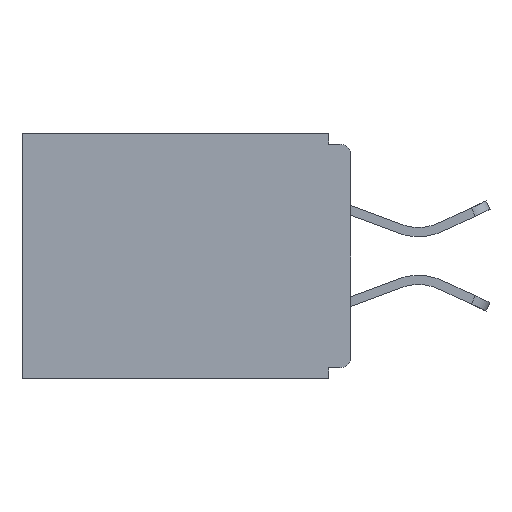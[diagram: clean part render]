
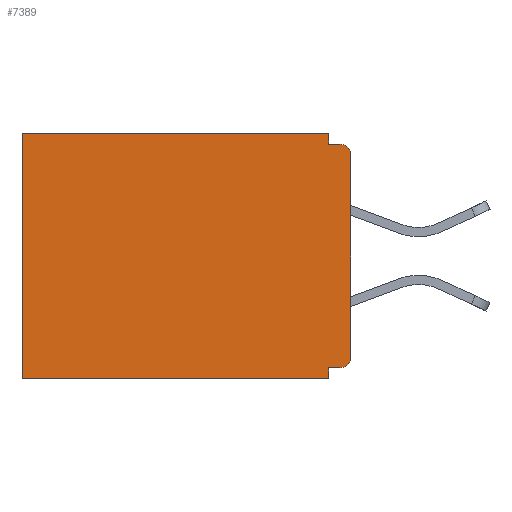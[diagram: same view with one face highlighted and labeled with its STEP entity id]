
A CAD part, left-side view. The second image highlights one B-rep face of the part: STEP entity #7389.
In plain terms, the highlighted planar face has unit normal (-1, 0, 0).
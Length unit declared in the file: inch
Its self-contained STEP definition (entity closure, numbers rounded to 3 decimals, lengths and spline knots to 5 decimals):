
#33 = ORIENTED_EDGE ( 'NONE', *, *, #11274, .F. ) ;
#66 = VECTOR ( 'NONE', #2666, 39.37008 ) ;
#391 = LINE ( 'NONE', #12094, #10864 ) ;
#463 = VECTOR ( 'NONE', #8896, 39.37008 ) ;
#676 = VERTEX_POINT ( 'NONE', #4409 ) ;
#1182 = VECTOR ( 'NONE', #12163, 39.37008 ) ;
#1606 = EDGE_CURVE ( 'NONE', #3405, #9363, #13358, .T. ) ;
#1811 = VECTOR ( 'NONE', #3227, 39.37008 ) ;
#2247 = LINE ( 'NONE', #7688, #2940 ) ;
#2350 = LINE ( 'NONE', #8434, #66 ) ;
#2666 = DIRECTION ( 'NONE',  ( 0., 1., 0. ) ) ;
#2933 = VERTEX_POINT ( 'NONE', #11107 ) ;
#2940 = VECTOR ( 'NONE', #10080, 39.37008 ) ;
#2948 = VERTEX_POINT ( 'NONE', #11156 ) ;
#2964 = ORIENTED_EDGE ( 'NONE', *, *, #5777, .T. ) ;
#3064 = DIRECTION ( 'NONE',  ( -1., 0., 0. ) ) ;
#3100 = ORIENTED_EDGE ( 'NONE', *, *, #1606, .F. ) ;
#3113 = ORIENTED_EDGE ( 'NONE', *, *, #5109, .T. ) ;
#3227 = DIRECTION ( 'NONE',  ( 0., 0., -1. ) ) ;
#3266 = CIRCLE ( 'NONE', #5534, 0.015 ) ;
#3405 = VERTEX_POINT ( 'NONE', #8879 ) ;
#3455 = VECTOR ( 'NONE', #6481, 39.37008 ) ;
#4177 = CARTESIAN_POINT ( 'NONE',  ( 0.298, 0., -0.015 ) ) ;
#4213 = DIRECTION ( 'NONE',  ( 0., 0., -1. ) ) ;
#4240 = AXIS2_PLACEMENT_3D ( 'NONE', #8435, #9583, #4910 ) ;
#4270 = CARTESIAN_POINT ( 'NONE',  ( 0.298, 0.031, -0.343 ) ) ;
#4409 = CARTESIAN_POINT ( 'NONE',  ( 0.298, 0.031, -0.343 ) ) ;
#4434 = ORIENTED_EDGE ( 'NONE', *, *, #14666, .F. ) ;
#4571 = VERTEX_POINT ( 'NONE', #10166 ) ;
#4628 = FACE_OUTER_BOUND ( 'NONE', #9321, .T. ) ;
#4910 = DIRECTION ( 'NONE',  ( 0., 0., -1. ) ) ;
#5109 = EDGE_CURVE ( 'NONE', #2948, #9160, #5795, .T. ) ;
#5123 = CARTESIAN_POINT ( 'NONE',  ( 0.298, 0.46, 0. ) ) ;
#5504 = CARTESIAN_POINT ( 'NONE',  ( 0.298, 0., -0.313 ) ) ;
#5534 = AXIS2_PLACEMENT_3D ( 'NONE', #9932, #3064, #4213 ) ;
#5617 = EDGE_CURVE ( 'NONE', #10846, #2948, #6871, .T. ) ;
#5777 = EDGE_CURVE ( 'NONE', #13731, #9363, #3266, .T. ) ;
#5795 = LINE ( 'NONE', #5123, #13452 ) ;
#5915 = CARTESIAN_POINT ( 'NONE',  ( 0.298, 0.015, -0.328 ) ) ;
#6049 = AXIS2_PLACEMENT_3D ( 'NONE', #11070, #7735, #7685 ) ;
#6290 = DIRECTION ( 'NONE',  ( 0., 0., -1. ) ) ;
#6481 = DIRECTION ( 'NONE',  ( 0., 0., -1. ) ) ;
#6674 = PLANE ( 'NONE',  #6049 ) ;
#6854 = CARTESIAN_POINT ( 'NONE',  ( 0.298, 0.46, -0.343 ) ) ;
#6871 = LINE ( 'NONE', #8862, #463 ) ;
#7298 = EDGE_CURVE ( 'NONE', #3405, #11659, #10030, .T. ) ;
#7389 = ADVANCED_FACE ( 'NONE', ( #4628 ), #6674, .F. ) ;
#7685 = DIRECTION ( 'NONE',  ( 0., 0., -1. ) ) ;
#7688 = CARTESIAN_POINT ( 'NONE',  ( 0.298, 0.031, -0.343 ) ) ;
#7735 = DIRECTION ( 'NONE',  ( 1., 0., 0. ) ) ;
#8434 = CARTESIAN_POINT ( 'NONE',  ( 0.298, 0., -0.343 ) ) ;
#8435 = CARTESIAN_POINT ( 'NONE',  ( 0.298, 0.015, -0.03 ) ) ;
#8682 = LINE ( 'NONE', #4177, #1182 ) ;
#8862 = CARTESIAN_POINT ( 'NONE',  ( 0.298, 0., 0. ) ) ;
#8879 = CARTESIAN_POINT ( 'NONE',  ( 0.298, 0., -0.03 ) ) ;
#8896 = DIRECTION ( 'NONE',  ( 0., 1., 0. ) ) ;
#9084 = CARTESIAN_POINT ( 'NONE',  ( 0.298, 0.015, -0.015 ) ) ;
#9160 = VERTEX_POINT ( 'NONE', #6854 ) ;
#9215 = EDGE_CURVE ( 'NONE', #10846, #2933, #2247, .T. ) ;
#9218 = EDGE_CURVE ( 'NONE', #4571, #676, #12906, .T. ) ;
#9321 = EDGE_LOOP ( 'NONE', ( #13784, #4434, #13448, #12890, #3113, #33, #12110, #10987, #2964, #3100 ) ) ;
#9329 = CARTESIAN_POINT ( 'NONE',  ( 0.298, 0.031, 0. ) ) ;
#9363 = VERTEX_POINT ( 'NONE', #5504 ) ;
#9583 = DIRECTION ( 'NONE',  ( -1., 0., 0. ) ) ;
#9932 = CARTESIAN_POINT ( 'NONE',  ( 0.298, 0.015, -0.313 ) ) ;
#9950 = CARTESIAN_POINT ( 'NONE',  ( 0.298, 0., 0. ) ) ;
#10030 = CIRCLE ( 'NONE', #4240, 0.015 ) ;
#10080 = DIRECTION ( 'NONE',  ( 0., 0., -1. ) ) ;
#10166 = CARTESIAN_POINT ( 'NONE',  ( 0.298, 0.031, -0.328 ) ) ;
#10846 = VERTEX_POINT ( 'NONE', #9329 ) ;
#10864 = VECTOR ( 'NONE', #14084, 39.37008 ) ;
#10987 = ORIENTED_EDGE ( 'NONE', *, *, #13076, .F. ) ;
#11070 = CARTESIAN_POINT ( 'NONE',  ( 0.298, 0., 0. ) ) ;
#11107 = CARTESIAN_POINT ( 'NONE',  ( 0.298, 0.031, -0.015 ) ) ;
#11156 = CARTESIAN_POINT ( 'NONE',  ( 0.298, 0.46, 0. ) ) ;
#11274 = EDGE_CURVE ( 'NONE', #676, #9160, #2350, .T. ) ;
#11659 = VERTEX_POINT ( 'NONE', #9084 ) ;
#12094 = CARTESIAN_POINT ( 'NONE',  ( 0.298, 0., -0.328 ) ) ;
#12110 = ORIENTED_EDGE ( 'NONE', *, *, #9218, .F. ) ;
#12163 = DIRECTION ( 'NONE',  ( 0., -1., 0. ) ) ;
#12890 = ORIENTED_EDGE ( 'NONE', *, *, #5617, .T. ) ;
#12906 = LINE ( 'NONE', #4270, #3455 ) ;
#13076 = EDGE_CURVE ( 'NONE', #13731, #4571, #391, .T. ) ;
#13358 = LINE ( 'NONE', #9950, #1811 ) ;
#13448 = ORIENTED_EDGE ( 'NONE', *, *, #9215, .F. ) ;
#13452 = VECTOR ( 'NONE', #6290, 39.37008 ) ;
#13731 = VERTEX_POINT ( 'NONE', #5915 ) ;
#13784 = ORIENTED_EDGE ( 'NONE', *, *, #7298, .T. ) ;
#14084 = DIRECTION ( 'NONE',  ( 0., 1., 0. ) ) ;
#14666 = EDGE_CURVE ( 'NONE', #2933, #11659, #8682, .T. ) ;
